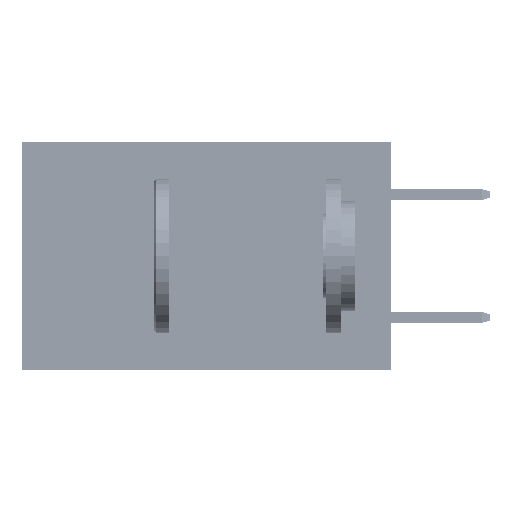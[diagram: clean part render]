
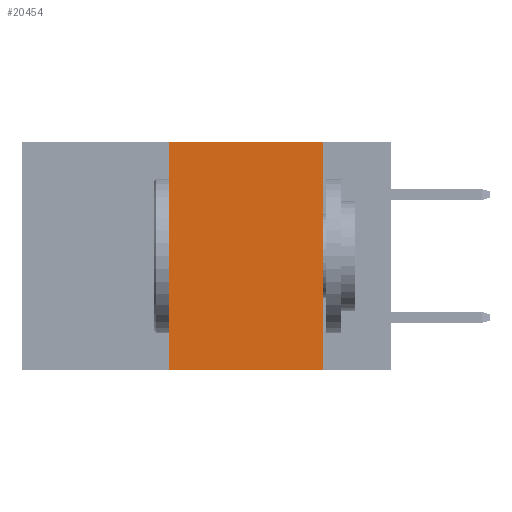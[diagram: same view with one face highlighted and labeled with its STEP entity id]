
A CAD part, left-side view. The second image highlights one B-rep face of the part: STEP entity #20454.
In plain terms, the highlighted planar face has unit normal (-1, 0, 0).
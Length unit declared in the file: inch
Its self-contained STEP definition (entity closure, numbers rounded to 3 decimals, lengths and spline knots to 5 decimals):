
#2002 = EDGE_CURVE ( 'NONE', #8207, #24973, #26244, .T. ) ;
#2456 = DIRECTION ( 'NONE',  ( 0., -1., 0. ) ) ;
#3652 = CARTESIAN_POINT ( 'NONE',  ( 0., 0.36, 0. ) ) ;
#3791 = DIRECTION ( 'NONE',  ( 1., 0., 0. ) ) ;
#4274 = DIRECTION ( 'NONE',  ( 0., 0., -1. ) ) ;
#4368 = VECTOR ( 'NONE', #17206, 39.37008 ) ;
#4838 = FACE_OUTER_BOUND ( 'NONE', #36670, .T. ) ;
#5198 = ORIENTED_EDGE ( 'NONE', *, *, #7965, .F. ) ;
#7965 = EDGE_CURVE ( 'NONE', #22370, #36751, #13779, .T. ) ;
#8207 = VERTEX_POINT ( 'NONE', #11930 ) ;
#11573 = ORIENTED_EDGE ( 'NONE', *, *, #18973, .F. ) ;
#11930 = CARTESIAN_POINT ( 'NONE',  ( 0., 0.36, -0.37 ) ) ;
#13779 = LINE ( 'NONE', #24928, #24686 ) ;
#14320 = CARTESIAN_POINT ( 'NONE',  ( 0., 0.11, 0. ) ) ;
#17064 = CARTESIAN_POINT ( 'NONE',  ( 0., 0.11, -0.37 ) ) ;
#17206 = DIRECTION ( 'NONE',  ( 0., 0., -1. ) ) ;
#17835 = CARTESIAN_POINT ( 'NONE',  ( 0., 0.6, -0.37 ) ) ;
#18973 = EDGE_CURVE ( 'NONE', #8207, #22370, #36429, .T. ) ;
#20454 = ADVANCED_FACE ( 'NONE', ( #4838 ), #29742, .F. ) ;
#20950 = VECTOR ( 'NONE', #32942, 39.37008 ) ;
#22370 = VERTEX_POINT ( 'NONE', #32742 ) ;
#22674 = CARTESIAN_POINT ( 'NONE',  ( 0., 0.6, 0. ) ) ;
#23840 = LINE ( 'NONE', #24271, #4368 ) ;
#24271 = CARTESIAN_POINT ( 'NONE',  ( 0., 0.11, 0. ) ) ;
#24686 = VECTOR ( 'NONE', #2456, 39.37008 ) ;
#24928 = CARTESIAN_POINT ( 'NONE',  ( 0., 0.6, 0. ) ) ;
#24973 = VERTEX_POINT ( 'NONE', #17064 ) ;
#26244 = LINE ( 'NONE', #17835, #46841 ) ;
#28737 = DIRECTION ( 'NONE',  ( 0., -1., 0. ) ) ;
#29742 = PLANE ( 'NONE',  #47471 ) ;
#32742 = CARTESIAN_POINT ( 'NONE',  ( 0., 0.36, 0. ) ) ;
#32942 = DIRECTION ( 'NONE',  ( 0., 0., 1. ) ) ;
#36429 = LINE ( 'NONE', #3652, #20950 ) ;
#36630 = EDGE_CURVE ( 'NONE', #36751, #24973, #23840, .T. ) ;
#36670 = EDGE_LOOP ( 'NONE', ( #46505, #5198, #11573, #41260 ) ) ;
#36751 = VERTEX_POINT ( 'NONE', #14320 ) ;
#41260 = ORIENTED_EDGE ( 'NONE', *, *, #2002, .T. ) ;
#46505 = ORIENTED_EDGE ( 'NONE', *, *, #36630, .F. ) ;
#46841 = VECTOR ( 'NONE', #28737, 39.37008 ) ;
#47471 = AXIS2_PLACEMENT_3D ( 'NONE', #22674, #3791, #4274 ) ;
